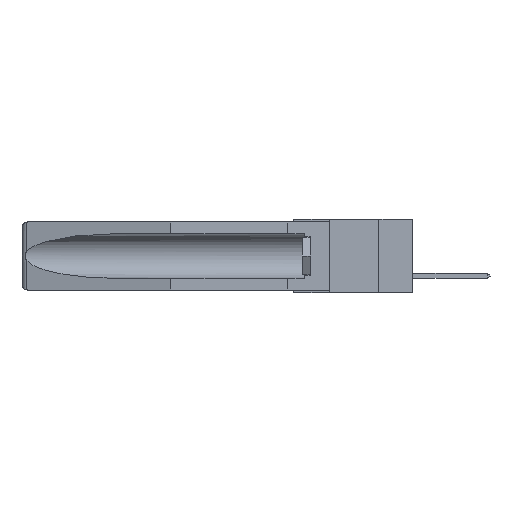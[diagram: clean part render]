
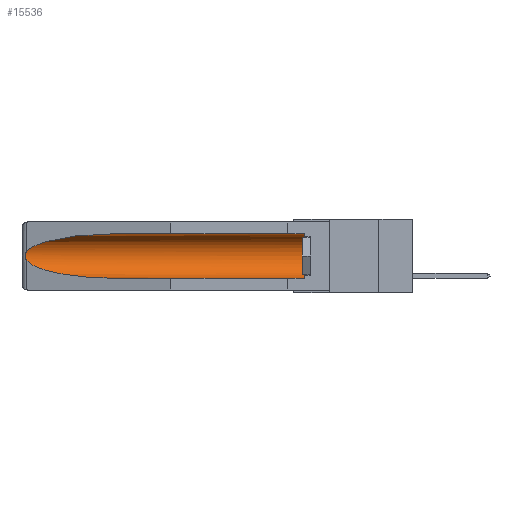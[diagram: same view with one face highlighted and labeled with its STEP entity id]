
A CAD part, left-side view. The second image highlights one B-rep face of the part: STEP entity #15536.
In plain terms, the highlighted cylindrical face has radius 2.857 mm (diameter 5.715 mm), a partial arc.
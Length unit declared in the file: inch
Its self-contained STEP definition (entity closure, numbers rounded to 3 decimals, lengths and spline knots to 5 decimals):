
#288 = EDGE_CURVE ( 'NONE', #13261, #938, #5418, .T. ) ;
#840 = CARTESIAN_POINT ( 'NONE',  ( 0.25451, 1.48313, -0.24835 ) ) ;
#854 = DIRECTION ( 'NONE',  ( 0., 0., 1. ) ) ;
#877 = CARTESIAN_POINT ( 'NONE',  ( 0.26597, 1.52961, -0.15275 ) ) ;
#930 = CARTESIAN_POINT ( 'NONE',  ( 0.2673, 1.5327, -0.16383 ) ) ;
#938 = VERTEX_POINT ( 'NONE', #10732 ) ;
#1004 = LINE ( 'NONE', #12113, #6628 ) ;
#1331 = DIRECTION ( 'NONE',  ( 0., 0., 1. ) ) ;
#2144 = CARTESIAN_POINT ( 'NONE',  ( 0.155, -0.30754, -0.1715 ) ) ;
#2166 = CARTESIAN_POINT ( 'NONE',  ( 0.26655, 1.53094, -0.18657 ) ) ;
#2220 = CARTESIAN_POINT ( 'NONE',  ( 0.26537, 1.52718, -0.14972 ) ) ;
#2400 = AXIS2_PLACEMENT_3D ( 'NONE', #2144, #12427, #854 ) ;
#2630 = DIRECTION ( 'NONE',  ( 0., 1., 0. ) ) ;
#2990 = AXIS2_PLACEMENT_3D ( 'NONE', #3749, #15307, #1331 ) ;
#3043 = ORIENTED_EDGE ( 'NONE', *, *, #288, .T. ) ;
#3229 = EDGE_CURVE ( 'NONE', #12899, #4632, #8934, .T. ) ;
#3280 = EDGE_LOOP ( 'NONE', ( #3043, #8883, #11566, #4853, #10849, #4341 ) ) ;
#3749 = CARTESIAN_POINT ( 'NONE',  ( 0.155, 0.126, -0.1715 ) ) ;
#4341 = ORIENTED_EDGE ( 'NONE', *, *, #10349, .T. ) ;
#4632 = VERTEX_POINT ( 'NONE', #11115 ) ;
#4798 = CARTESIAN_POINT ( 'NONE',  ( 0.2675, 1.53308, -0.17534 ) ) ;
#4804 = EDGE_CURVE ( 'NONE', #15643, #4632, #1004, .T. ) ;
#4853 = ORIENTED_EDGE ( 'NONE', *, *, #4804, .F. ) ;
#5418 =( BOUNDED_CURVE ( )  B_SPLINE_CURVE ( 3, ( #12985, #7809, #14318, #10288 ),
 .UNSPECIFIED., .F., .F. ) 
 B_SPLINE_CURVE_WITH_KNOTS ( ( 4, 4 ),
 ( 4.71239, 6.08839 ),
 .UNSPECIFIED. ) 
 CURVE ( )  GEOMETRIC_REPRESENTATION_ITEM ( )  RATIONAL_B_SPLINE_CURVE ( ( 1., 0.848, 0.848, 1. ) ) 
 REPRESENTATION_ITEM ( '' )  );
#5551 = LINE ( 'NONE', #9100, #12808 ) ;
#5822 = B_SPLINE_CURVE_WITH_KNOTS ( 'NONE', 3,
 ( #2220, #877, #11040, #930, #9859, #4798, #16202, #2166, #9696, #10983 ),
 .UNSPECIFIED., .F., .F.,
 ( 4, 2, 2, 2, 4 ),
 ( 0., 0.00029, 0.00058, 0.00087, 0.00117 ),
 .UNSPECIFIED. ) ;
#6176 = CARTESIAN_POINT ( 'NONE',  ( 0.155, 0.126, -0.284 ) ) ;
#6628 = VECTOR ( 'NONE', #16201, 39.37008 ) ;
#6807 = CIRCLE ( 'NONE', #2990, 0.1125 ) ;
#7809 = CARTESIAN_POINT ( 'NONE',  ( 0.21114, 1.30732, -0.059 ) ) ;
#8110 = CYLINDRICAL_SURFACE ( 'NONE', #2400, 0.1125 ) ;
#8883 = ORIENTED_EDGE ( 'NONE', *, *, #12800, .T. ) ;
#8934 =( BOUNDED_CURVE ( )  B_SPLINE_CURVE ( 3, ( #16171, #840, #13695, #15254 ),
 .UNSPECIFIED., .F., .F. ) 
 B_SPLINE_CURVE_WITH_KNOTS ( ( 4, 4 ),
 ( 0.1948, 1.5708 ),
 .UNSPECIFIED. ) 
 CURVE ( )  GEOMETRIC_REPRESENTATION_ITEM ( )  RATIONAL_B_SPLINE_CURVE ( ( 1., 0.848, 0.848, 1. ) ) 
 REPRESENTATION_ITEM ( '' )  );
#9100 = CARTESIAN_POINT ( 'NONE',  ( 0.155, -0.30754, -0.059 ) ) ;
#9688 = EDGE_CURVE ( 'NONE', #15643, #14880, #6807, .T. ) ;
#9696 = CARTESIAN_POINT ( 'NONE',  ( 0.26597, 1.5296, -0.19026 ) ) ;
#9859 = CARTESIAN_POINT ( 'NONE',  ( 0.2675, 1.53308, -0.16763 ) ) ;
#10265 = CARTESIAN_POINT ( 'NONE',  ( 0.155, 0.126, -0.059 ) ) ;
#10288 = CARTESIAN_POINT ( 'NONE',  ( 0.26537, 1.52718, -0.14972 ) ) ;
#10349 = EDGE_CURVE ( 'NONE', #14880, #13261, #5551, .T. ) ;
#10732 = CARTESIAN_POINT ( 'NONE',  ( 0.26537, 1.52718, -0.14972 ) ) ;
#10843 = CARTESIAN_POINT ( 'NONE',  ( 0.155, 1.07973, -0.059 ) ) ;
#10849 = ORIENTED_EDGE ( 'NONE', *, *, #9688, .T. ) ;
#10983 = CARTESIAN_POINT ( 'NONE',  ( 0.26537, 1.52718, -0.19328 ) ) ;
#11040 = CARTESIAN_POINT ( 'NONE',  ( 0.26654, 1.53092, -0.15636 ) ) ;
#11115 = CARTESIAN_POINT ( 'NONE',  ( 0.155, 1.07973, -0.284 ) ) ;
#11521 = FACE_OUTER_BOUND ( 'NONE', #3280, .T. ) ;
#11566 = ORIENTED_EDGE ( 'NONE', *, *, #3229, .T. ) ;
#12113 = CARTESIAN_POINT ( 'NONE',  ( 0.155, -0.30754, -0.284 ) ) ;
#12427 = DIRECTION ( 'NONE',  ( 0., 1., 0. ) ) ;
#12800 = EDGE_CURVE ( 'NONE', #938, #12899, #5822, .T. ) ;
#12808 = VECTOR ( 'NONE', #2630, 39.37008 ) ;
#12899 = VERTEX_POINT ( 'NONE', #13836 ) ;
#12985 = CARTESIAN_POINT ( 'NONE',  ( 0.155, 1.07973, -0.059 ) ) ;
#13261 = VERTEX_POINT ( 'NONE', #10843 ) ;
#13695 = CARTESIAN_POINT ( 'NONE',  ( 0.21114, 1.30732, -0.284 ) ) ;
#13836 = CARTESIAN_POINT ( 'NONE',  ( 0.26537, 1.52718, -0.19328 ) ) ;
#14318 = CARTESIAN_POINT ( 'NONE',  ( 0.25451, 1.48313, -0.09465 ) ) ;
#14880 = VERTEX_POINT ( 'NONE', #10265 ) ;
#15254 = CARTESIAN_POINT ( 'NONE',  ( 0.155, 1.07973, -0.284 ) ) ;
#15307 = DIRECTION ( 'NONE',  ( 0., -1., 0. ) ) ;
#15536 = ADVANCED_FACE ( 'NONE', ( #11521 ), #8110, .F. ) ;
#15643 = VERTEX_POINT ( 'NONE', #6176 ) ;
#16171 = CARTESIAN_POINT ( 'NONE',  ( 0.26537, 1.52718, -0.19328 ) ) ;
#16201 = DIRECTION ( 'NONE',  ( 0., 1., 0. ) ) ;
#16202 = CARTESIAN_POINT ( 'NONE',  ( 0.2673, 1.53269, -0.17917 ) ) ;
